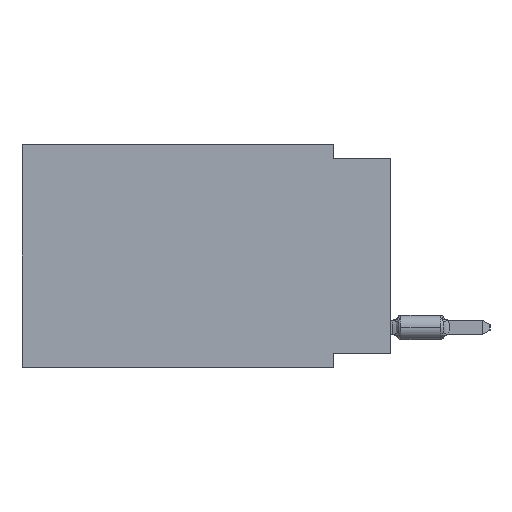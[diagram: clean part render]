
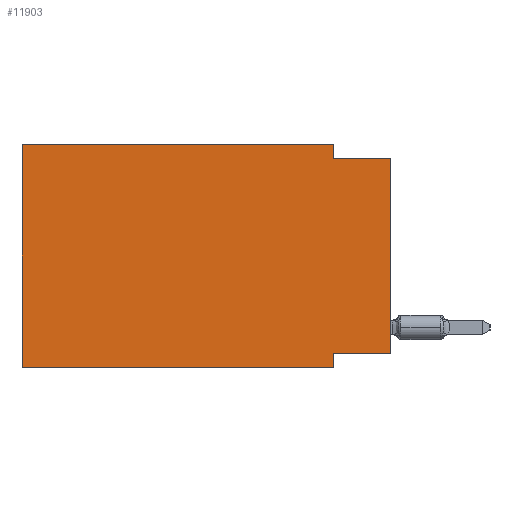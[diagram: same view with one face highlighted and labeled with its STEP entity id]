
A CAD part, left-side view. The second image highlights one B-rep face of the part: STEP entity #11903.
In plain terms, the highlighted planar face has unit normal (-1, 0, 0).
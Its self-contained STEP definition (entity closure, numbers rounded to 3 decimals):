
#587 = VECTOR ( 'NONE', #14860, 1000. ) ;
#1847 = PLANE ( 'NONE',  #25075 ) ;
#2492 = LINE ( 'NONE', #40531, #21412 ) ;
#4936 = EDGE_CURVE ( 'NONE', #24819, #31160, #64495, .T. ) ;
#6597 = ORIENTED_EDGE ( 'NONE', *, *, #24549, .F. ) ;
#6762 = CARTESIAN_POINT ( 'NONE',  ( 0., 2.54, -9.271 ) ) ;
#6893 = LINE ( 'NONE', #58908, #38569 ) ;
#7529 = CARTESIAN_POINT ( 'NONE',  ( 0., 16.383, 0. ) ) ;
#8016 = CARTESIAN_POINT ( 'NONE',  ( 0., 0., -9.271 ) ) ;
#8572 = ORIENTED_EDGE ( 'NONE', *, *, #4936, .F. ) ;
#10144 = VECTOR ( 'NONE', #14373, 1000. ) ;
#11701 = CARTESIAN_POINT ( 'NONE',  ( 0., 16.383, -9.906 ) ) ;
#11903 = ADVANCED_FACE ( 'NONE', ( #49668 ), #1847, .F. ) ;
#12106 = CARTESIAN_POINT ( 'NONE',  ( 0., 2.54, -0.635 ) ) ;
#13427 = VECTOR ( 'NONE', #23167, 1000. ) ;
#13534 = ORIENTED_EDGE ( 'NONE', *, *, #43139, .T. ) ;
#14373 = DIRECTION ( 'NONE',  ( 0., 0., -1. ) ) ;
#14860 = DIRECTION ( 'NONE',  ( 0., -1., 0. ) ) ;
#16330 = CARTESIAN_POINT ( 'NONE',  ( 0., 16.383, 0. ) ) ;
#18007 = EDGE_CURVE ( 'NONE', #39563, #56187, #48297, .T. ) ;
#18033 = VERTEX_POINT ( 'NONE', #22486 ) ;
#21412 = VECTOR ( 'NONE', #30063, 1000. ) ;
#22017 = EDGE_CURVE ( 'NONE', #52264, #39563, #6893, .T. ) ;
#22486 = CARTESIAN_POINT ( 'NONE',  ( 0., 16.383, -9.906 ) ) ;
#23167 = DIRECTION ( 'NONE',  ( 0., 0., -1. ) ) ;
#23171 = CARTESIAN_POINT ( 'NONE',  ( 0., 16.383, 0. ) ) ;
#23936 = CARTESIAN_POINT ( 'NONE',  ( 0., 2.54, -9.906 ) ) ;
#24549 = EDGE_CURVE ( 'NONE', #31160, #34760, #41226, .T. ) ;
#24819 = VERTEX_POINT ( 'NONE', #16330 ) ;
#25075 = AXIS2_PLACEMENT_3D ( 'NONE', #23171, #44432, #39520 ) ;
#25265 = EDGE_CURVE ( 'NONE', #52264, #40241, #2492, .T. ) ;
#27362 = CARTESIAN_POINT ( 'NONE',  ( 0., 2.54, -9.906 ) ) ;
#27701 = EDGE_CURVE ( 'NONE', #18033, #24819, #38293, .T. ) ;
#30063 = DIRECTION ( 'NONE',  ( 0., 0., 1. ) ) ;
#31160 = VERTEX_POINT ( 'NONE', #67759 ) ;
#31406 = CARTESIAN_POINT ( 'NONE',  ( 0., 16.383, 0. ) ) ;
#34268 = ORIENTED_EDGE ( 'NONE', *, *, #25265, .T. ) ;
#34760 = VERTEX_POINT ( 'NONE', #12106 ) ;
#34968 = EDGE_CURVE ( 'NONE', #34760, #40241, #41037, .T. ) ;
#36992 = DIRECTION ( 'NONE',  ( 0., -1., 0. ) ) ;
#38293 = LINE ( 'NONE', #7529, #57541 ) ;
#38569 = VECTOR ( 'NONE', #38645, 1000. ) ;
#38645 = DIRECTION ( 'NONE',  ( 0., 1., 0. ) ) ;
#39520 = DIRECTION ( 'NONE',  ( 0., 0., -1. ) ) ;
#39563 = VERTEX_POINT ( 'NONE', #6762 ) ;
#40241 = VERTEX_POINT ( 'NONE', #43062 ) ;
#40531 = CARTESIAN_POINT ( 'NONE',  ( 0., 0., 0. ) ) ;
#41037 = LINE ( 'NONE', #62630, #587 ) ;
#41073 = VECTOR ( 'NONE', #36992, 1000. ) ;
#41226 = LINE ( 'NONE', #62818, #10144 ) ;
#42027 = VECTOR ( 'NONE', #54275, 1000. ) ;
#43062 = CARTESIAN_POINT ( 'NONE',  ( 0., 0., -0.635 ) ) ;
#43139 = EDGE_CURVE ( 'NONE', #18033, #56187, #59496, .T. ) ;
#44252 = ORIENTED_EDGE ( 'NONE', *, *, #18007, .F. ) ;
#44432 = DIRECTION ( 'NONE',  ( 1., 0., 0. ) ) ;
#48297 = LINE ( 'NONE', #27362, #13427 ) ;
#49668 = FACE_OUTER_BOUND ( 'NONE', #54477, .T. ) ;
#50719 = ORIENTED_EDGE ( 'NONE', *, *, #27701, .F. ) ;
#51302 = ORIENTED_EDGE ( 'NONE', *, *, #34968, .F. ) ;
#52264 = VERTEX_POINT ( 'NONE', #8016 ) ;
#54275 = DIRECTION ( 'NONE',  ( 0., -1., 0. ) ) ;
#54477 = EDGE_LOOP ( 'NONE', ( #34268, #51302, #6597, #8572, #50719, #13534, #44252, #59144 ) ) ;
#55034 = DIRECTION ( 'NONE',  ( 0., 0., 1. ) ) ;
#56187 = VERTEX_POINT ( 'NONE', #23936 ) ;
#57541 = VECTOR ( 'NONE', #55034, 1000. ) ;
#58908 = CARTESIAN_POINT ( 'NONE',  ( 0., 0., -9.271 ) ) ;
#59144 = ORIENTED_EDGE ( 'NONE', *, *, #22017, .F. ) ;
#59496 = LINE ( 'NONE', #11701, #42027 ) ;
#62630 = CARTESIAN_POINT ( 'NONE',  ( 0., 0., -0.635 ) ) ;
#62818 = CARTESIAN_POINT ( 'NONE',  ( 0., 2.54, 0. ) ) ;
#64495 = LINE ( 'NONE', #31406, #41073 ) ;
#67759 = CARTESIAN_POINT ( 'NONE',  ( 0., 2.54, 0. ) ) ;
